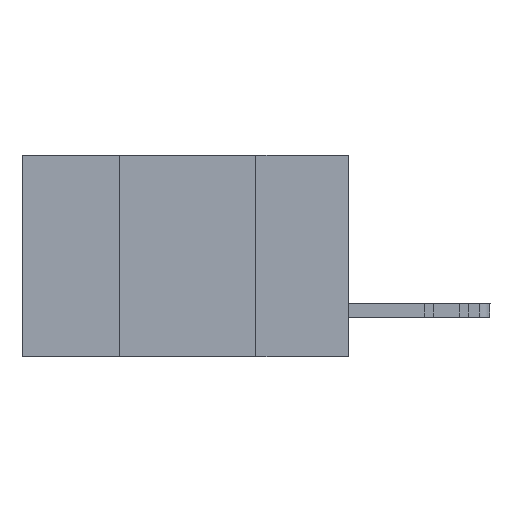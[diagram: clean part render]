
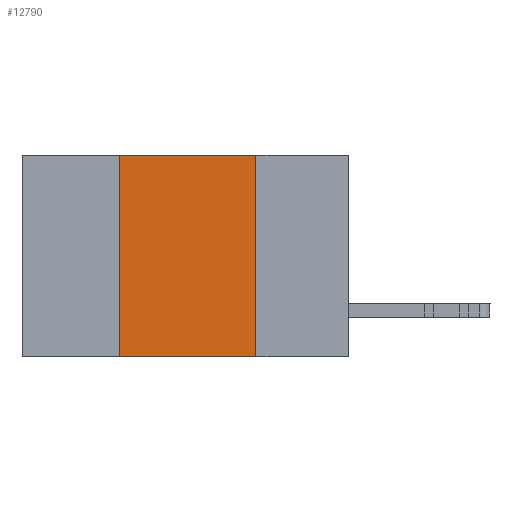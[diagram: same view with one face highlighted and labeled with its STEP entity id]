
A CAD part, left-side view. The second image highlights one B-rep face of the part: STEP entity #12790.
In plain terms, the highlighted planar face has unit normal (-1, 0, 0).
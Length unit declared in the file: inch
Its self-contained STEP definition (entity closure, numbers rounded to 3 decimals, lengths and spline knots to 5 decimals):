
#91 = EDGE_CURVE ( 'NONE', #1553, #20380, #10776, .T. ) ;
#1553 = VERTEX_POINT ( 'NONE', #9771 ) ;
#3528 = EDGE_LOOP ( 'NONE', ( #19479, #15438, #23144, #7872 ) ) ;
#5369 = VERTEX_POINT ( 'NONE', #12941 ) ;
#5973 = DIRECTION ( 'NONE',  ( 0., 0., -1. ) ) ;
#6218 = DIRECTION ( 'NONE',  ( 1., 0., 0. ) ) ;
#6294 = CARTESIAN_POINT ( 'NONE',  ( 0., 0.6, 0. ) ) ;
#6417 = PLANE ( 'NONE',  #20436 ) ;
#6570 = EDGE_CURVE ( 'NONE', #15155, #20380, #11758, .T. ) ;
#7872 = ORIENTED_EDGE ( 'NONE', *, *, #6570, .T. ) ;
#8292 = FACE_OUTER_BOUND ( 'NONE', #3528, .T. ) ;
#8868 = LINE ( 'NONE', #11351, #9504 ) ;
#9504 = VECTOR ( 'NONE', #25152, 39.37008 ) ;
#9771 = CARTESIAN_POINT ( 'NONE',  ( 0., 0.17, 0. ) ) ;
#9902 = LINE ( 'NONE', #22850, #15257 ) ;
#10776 = LINE ( 'NONE', #22627, #20753 ) ;
#10959 = DIRECTION ( 'NONE',  ( 0., -1., 0. ) ) ;
#11351 = CARTESIAN_POINT ( 'NONE',  ( 0., 0.42, -0.37 ) ) ;
#11758 = LINE ( 'NONE', #17366, #16482 ) ;
#12790 = ADVANCED_FACE ( 'NONE', ( #8292 ), #6417, .F. ) ;
#12941 = CARTESIAN_POINT ( 'NONE',  ( 0., 0.42, 0. ) ) ;
#15155 = VERTEX_POINT ( 'NONE', #18050 ) ;
#15257 = VECTOR ( 'NONE', #10959, 39.37008 ) ;
#15438 = ORIENTED_EDGE ( 'NONE', *, *, #21528, .F. ) ;
#16482 = VECTOR ( 'NONE', #17448, 39.37008 ) ;
#17366 = CARTESIAN_POINT ( 'NONE',  ( 0., 0.6, -0.37 ) ) ;
#17448 = DIRECTION ( 'NONE',  ( 0., -1., 0. ) ) ;
#17685 = EDGE_CURVE ( 'NONE', #15155, #5369, #8868, .T. ) ;
#18050 = CARTESIAN_POINT ( 'NONE',  ( 0., 0.42, -0.37 ) ) ;
#19479 = ORIENTED_EDGE ( 'NONE', *, *, #91, .F. ) ;
#20380 = VERTEX_POINT ( 'NONE', #22895 ) ;
#20436 = AXIS2_PLACEMENT_3D ( 'NONE', #6294, #6218, #5973 ) ;
#20753 = VECTOR ( 'NONE', #21758, 39.37008 ) ;
#21528 = EDGE_CURVE ( 'NONE', #5369, #1553, #9902, .T. ) ;
#21758 = DIRECTION ( 'NONE',  ( 0., 0., -1. ) ) ;
#22627 = CARTESIAN_POINT ( 'NONE',  ( 0., 0.17, -0.37 ) ) ;
#22850 = CARTESIAN_POINT ( 'NONE',  ( 0., 0.6, 0. ) ) ;
#22895 = CARTESIAN_POINT ( 'NONE',  ( 0., 0.17, -0.37 ) ) ;
#23144 = ORIENTED_EDGE ( 'NONE', *, *, #17685, .F. ) ;
#25152 = DIRECTION ( 'NONE',  ( 0., 0., 1. ) ) ;
